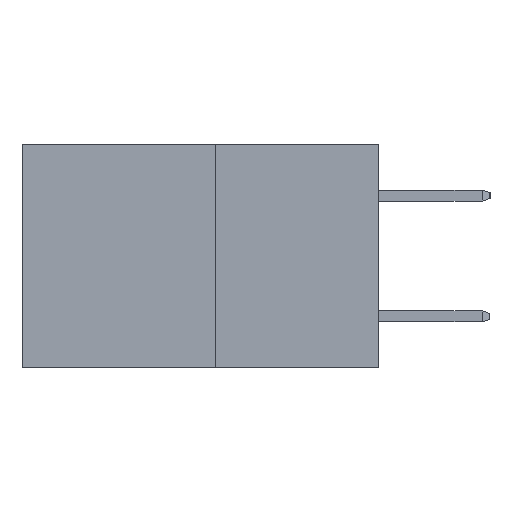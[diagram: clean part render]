
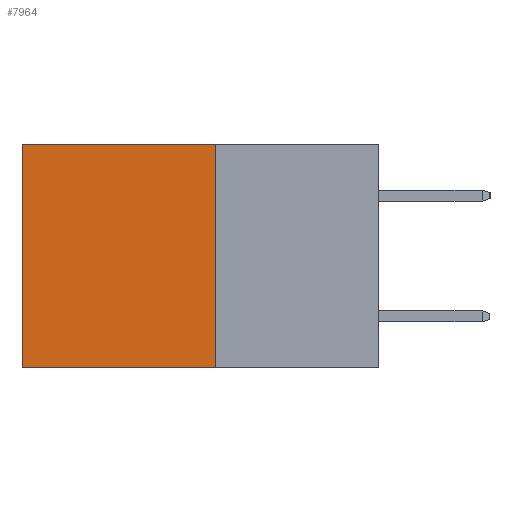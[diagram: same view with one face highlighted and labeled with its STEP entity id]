
A CAD part, left-side view. The second image highlights one B-rep face of the part: STEP entity #7964.
In plain terms, the highlighted planar face has unit normal (-1, 0, 0).
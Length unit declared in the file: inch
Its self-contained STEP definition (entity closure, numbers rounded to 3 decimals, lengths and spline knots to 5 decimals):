
#470 = CARTESIAN_POINT ( 'NONE',  ( 0.277, 0.59, -0.37 ) ) ;
#531 = CARTESIAN_POINT ( 'NONE',  ( 0.277, 0.59, -0.37 ) ) ;
#604 = EDGE_CURVE ( 'NONE', #10791, #4219, #2978, .T. ) ;
#1092 = PLANE ( 'NONE',  #5715 ) ;
#1833 = VERTEX_POINT ( 'NONE', #531 ) ;
#1968 = CARTESIAN_POINT ( 'NONE',  ( 0.277, 0.27, -0.37 ) ) ;
#2124 = FACE_OUTER_BOUND ( 'NONE', #2804, .T. ) ;
#2417 = VERTEX_POINT ( 'NONE', #7866 ) ;
#2602 = ORIENTED_EDGE ( 'NONE', *, *, #604, .T. ) ;
#2804 = EDGE_LOOP ( 'NONE', ( #6071, #10935, #10407, #2602 ) ) ;
#2978 = LINE ( 'NONE', #13691, #6507 ) ;
#3664 = DIRECTION ( 'NONE',  ( 1., 0., 0. ) ) ;
#4219 = VERTEX_POINT ( 'NONE', #8014 ) ;
#4322 = DIRECTION ( 'NONE',  ( 0., 0., -1. ) ) ;
#5229 = VECTOR ( 'NONE', #9708, 39.37008 ) ;
#5307 = EDGE_CURVE ( 'NONE', #4219, #1833, #7603, .T. ) ;
#5366 = DIRECTION ( 'NONE',  ( 0., 1., 0. ) ) ;
#5392 = EDGE_CURVE ( 'NONE', #2417, #1833, #14734, .T. ) ;
#5715 = AXIS2_PLACEMENT_3D ( 'NONE', #11253, #3664, #12415 ) ;
#6071 = ORIENTED_EDGE ( 'NONE', *, *, #5307, .T. ) ;
#6507 = VECTOR ( 'NONE', #5366, 39.37008 ) ;
#7171 = EDGE_CURVE ( 'NONE', #10791, #2417, #8280, .T. ) ;
#7603 = LINE ( 'NONE', #470, #10839 ) ;
#7866 = CARTESIAN_POINT ( 'NONE',  ( 0.277, 0.27, -0.37 ) ) ;
#7964 = ADVANCED_FACE ( 'NONE', ( #2124 ), #1092, .F. ) ;
#8014 = CARTESIAN_POINT ( 'NONE',  ( 0.277, 0.59, 0. ) ) ;
#8280 = LINE ( 'NONE', #1968, #5229 ) ;
#9708 = DIRECTION ( 'NONE',  ( 0., 0., -1. ) ) ;
#10407 = ORIENTED_EDGE ( 'NONE', *, *, #7171, .F. ) ;
#10791 = VERTEX_POINT ( 'NONE', #11363 ) ;
#10839 = VECTOR ( 'NONE', #4322, 39.37008 ) ;
#10935 = ORIENTED_EDGE ( 'NONE', *, *, #5392, .F. ) ;
#11253 = CARTESIAN_POINT ( 'NONE',  ( 0.277, 0.27, -0.37 ) ) ;
#11363 = CARTESIAN_POINT ( 'NONE',  ( 0.277, 0.27, 0. ) ) ;
#11715 = VECTOR ( 'NONE', #15383, 39.37008 ) ;
#12415 = DIRECTION ( 'NONE',  ( 0., 0., -1. ) ) ;
#13691 = CARTESIAN_POINT ( 'NONE',  ( 0.277, 0.27, 0. ) ) ;
#14734 = LINE ( 'NONE', #15426, #11715 ) ;
#15383 = DIRECTION ( 'NONE',  ( 0., 1., 0. ) ) ;
#15426 = CARTESIAN_POINT ( 'NONE',  ( 0.277, 0.27, -0.37 ) ) ;
